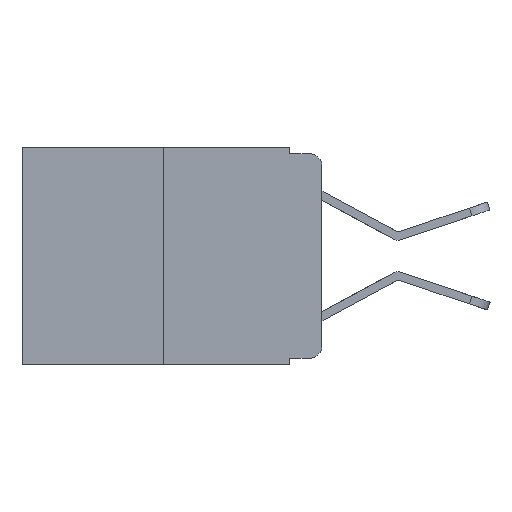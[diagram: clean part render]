
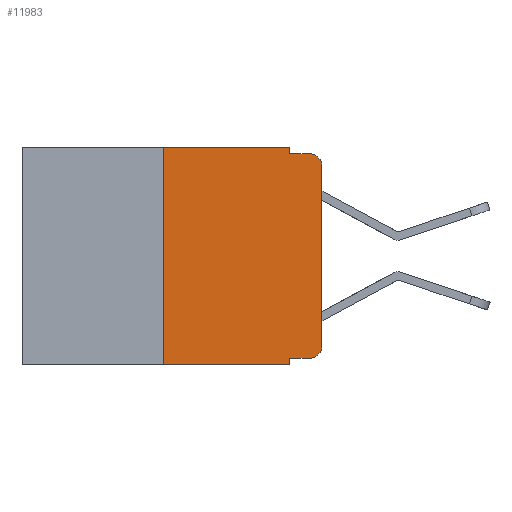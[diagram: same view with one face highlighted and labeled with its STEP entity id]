
A CAD part, left-side view. The second image highlights one B-rep face of the part: STEP entity #11983.
In plain terms, the highlighted planar face has unit normal (-1, 0, 0).
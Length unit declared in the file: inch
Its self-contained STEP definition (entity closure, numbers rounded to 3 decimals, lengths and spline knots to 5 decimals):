
#173 = DIRECTION ( 'NONE',  ( 0., -1., 0. ) ) ;
#198 = VECTOR ( 'NONE', #380, 39.37008 ) ;
#200 = LINE ( 'NONE', #7960, #8221 ) ;
#313 = AXIS2_PLACEMENT_3D ( 'NONE', #4580, #5464, #7419 ) ;
#380 = DIRECTION ( 'NONE',  ( 0., 0., 1. ) ) ;
#635 = CARTESIAN_POINT ( 'NONE',  ( 0., 0.051, 0. ) ) ;
#822 = EDGE_CURVE ( 'NONE', #8883, #10150, #1098, .T. ) ;
#1098 = CIRCLE ( 'NONE', #313, 0.02 ) ;
#1242 = DIRECTION ( 'NONE',  ( 0., -1., 0. ) ) ;
#1503 = DIRECTION ( 'NONE',  ( 0., 0., -1. ) ) ;
#2232 = VECTOR ( 'NONE', #1503, 39.37008 ) ;
#2392 = LINE ( 'NONE', #9920, #5976 ) ;
#2397 = VECTOR ( 'NONE', #3632, 39.37008 ) ;
#3114 = CARTESIAN_POINT ( 'NONE',  ( 0., 0.473, 0. ) ) ;
#3235 = PLANE ( 'NONE',  #10564 ) ;
#3454 = ORIENTED_EDGE ( 'NONE', *, *, #11480, .T. ) ;
#3479 = EDGE_LOOP ( 'NONE', ( #3454, #9024, #11172, #4703, #6198, #9509, #5245, #9219, #12142, #6382 ) ) ;
#3632 = DIRECTION ( 'NONE',  ( 0., -1., 0. ) ) ;
#3777 = VECTOR ( 'NONE', #173, 39.37008 ) ;
#3817 = CARTESIAN_POINT ( 'NONE',  ( 0., 0.25, 0. ) ) ;
#3969 = CARTESIAN_POINT ( 'NONE',  ( 0., 0.051, -0.01 ) ) ;
#4096 = CARTESIAN_POINT ( 'NONE',  ( 0., 0.02, -0.01 ) ) ;
#4369 = VECTOR ( 'NONE', #1242, 39.37008 ) ;
#4471 = EDGE_CURVE ( 'NONE', #8700, #10573, #9124, .T. ) ;
#4580 = CARTESIAN_POINT ( 'NONE',  ( 0., 0.02, -0.03 ) ) ;
#4703 = ORIENTED_EDGE ( 'NONE', *, *, #4769, .F. ) ;
#4769 = EDGE_CURVE ( 'NONE', #6133, #11857, #11927, .T. ) ;
#4968 = CARTESIAN_POINT ( 'NONE',  ( 0., 0.051, -0.333 ) ) ;
#5025 = VERTEX_POINT ( 'NONE', #10648 ) ;
#5245 = ORIENTED_EDGE ( 'NONE', *, *, #10837, .T. ) ;
#5464 = DIRECTION ( 'NONE',  ( -1., 0., 0. ) ) ;
#5537 = VERTEX_POINT ( 'NONE', #10692 ) ;
#5610 = LINE ( 'NONE', #11385, #2397 ) ;
#5696 = VECTOR ( 'NONE', #7408, 39.37008 ) ;
#5976 = VECTOR ( 'NONE', #8964, 39.37008 ) ;
#6019 = DIRECTION ( 'NONE',  ( 0., 0., -1. ) ) ;
#6133 = VERTEX_POINT ( 'NONE', #9936 ) ;
#6198 = ORIENTED_EDGE ( 'NONE', *, *, #11850, .F. ) ;
#6331 = AXIS2_PLACEMENT_3D ( 'NONE', #10434, #12134, #12237 ) ;
#6382 = ORIENTED_EDGE ( 'NONE', *, *, #4471, .T. ) ;
#6521 = EDGE_CURVE ( 'NONE', #5025, #9611, #2392, .T. ) ;
#6592 = LINE ( 'NONE', #6724, #5696 ) ;
#6626 = CARTESIAN_POINT ( 'NONE',  ( 0., 0.473, 0. ) ) ;
#6724 = CARTESIAN_POINT ( 'NONE',  ( 0., 0.051, -0.01 ) ) ;
#6793 = CARTESIAN_POINT ( 'NONE',  ( 0., 0., -0.313 ) ) ;
#7153 = EDGE_CURVE ( 'NONE', #5537, #9180, #200, .T. ) ;
#7204 = LINE ( 'NONE', #9925, #198 ) ;
#7408 = DIRECTION ( 'NONE',  ( 0., -1., 0. ) ) ;
#7419 = DIRECTION ( 'NONE',  ( 0., 0., -1. ) ) ;
#7775 = DIRECTION ( 'NONE',  ( 0., 0., 1. ) ) ;
#7869 = FACE_OUTER_BOUND ( 'NONE', #3479, .T. ) ;
#7960 = CARTESIAN_POINT ( 'NONE',  ( 0., 0.25, 0. ) ) ;
#8221 = VECTOR ( 'NONE', #7775, 39.37008 ) ;
#8575 = CARTESIAN_POINT ( 'NONE',  ( 0., 0.051, -0.343 ) ) ;
#8700 = VERTEX_POINT ( 'NONE', #12201 ) ;
#8883 = VERTEX_POINT ( 'NONE', #9890 ) ;
#8964 = DIRECTION ( 'NONE',  ( 0., 0., -1. ) ) ;
#9024 = ORIENTED_EDGE ( 'NONE', *, *, #822, .T. ) ;
#9124 = CIRCLE ( 'NONE', #6331, 0.02 ) ;
#9179 = EDGE_CURVE ( 'NONE', #11857, #10150, #6592, .T. ) ;
#9180 = VERTEX_POINT ( 'NONE', #3817 ) ;
#9219 = ORIENTED_EDGE ( 'NONE', *, *, #6521, .F. ) ;
#9509 = ORIENTED_EDGE ( 'NONE', *, *, #7153, .F. ) ;
#9611 = VERTEX_POINT ( 'NONE', #8575 ) ;
#9890 = CARTESIAN_POINT ( 'NONE',  ( 0., 0., -0.03 ) ) ;
#9920 = CARTESIAN_POINT ( 'NONE',  ( 0., 0.051, 0. ) ) ;
#9925 = CARTESIAN_POINT ( 'NONE',  ( 0., 0., 0. ) ) ;
#9936 = CARTESIAN_POINT ( 'NONE',  ( 0., 0.051, 0. ) ) ;
#10150 = VERTEX_POINT ( 'NONE', #4096 ) ;
#10434 = CARTESIAN_POINT ( 'NONE',  ( 0., 0.02, -0.313 ) ) ;
#10464 = LINE ( 'NONE', #6626, #3777 ) ;
#10564 = AXIS2_PLACEMENT_3D ( 'NONE', #3114, #10831, #6019 ) ;
#10573 = VERTEX_POINT ( 'NONE', #6793 ) ;
#10648 = CARTESIAN_POINT ( 'NONE',  ( 0., 0.051, -0.333 ) ) ;
#10692 = CARTESIAN_POINT ( 'NONE',  ( 0., 0.25, -0.343 ) ) ;
#10831 = DIRECTION ( 'NONE',  ( 1., 0., 0. ) ) ;
#10837 = EDGE_CURVE ( 'NONE', #5537, #9611, #5610, .T. ) ;
#11172 = ORIENTED_EDGE ( 'NONE', *, *, #9179, .F. ) ;
#11267 = EDGE_CURVE ( 'NONE', #5025, #8700, #11660, .T. ) ;
#11385 = CARTESIAN_POINT ( 'NONE',  ( 0., 0.473, -0.343 ) ) ;
#11480 = EDGE_CURVE ( 'NONE', #10573, #8883, #7204, .T. ) ;
#11660 = LINE ( 'NONE', #4968, #4369 ) ;
#11850 = EDGE_CURVE ( 'NONE', #9180, #6133, #10464, .T. ) ;
#11857 = VERTEX_POINT ( 'NONE', #3969 ) ;
#11927 = LINE ( 'NONE', #635, #2232 ) ;
#11983 = ADVANCED_FACE ( 'NONE', ( #7869 ), #3235, .F. ) ;
#12134 = DIRECTION ( 'NONE',  ( -1., 0., 0. ) ) ;
#12142 = ORIENTED_EDGE ( 'NONE', *, *, #11267, .T. ) ;
#12201 = CARTESIAN_POINT ( 'NONE',  ( 0., 0.02, -0.333 ) ) ;
#12237 = DIRECTION ( 'NONE',  ( 0., 0., -1. ) ) ;
